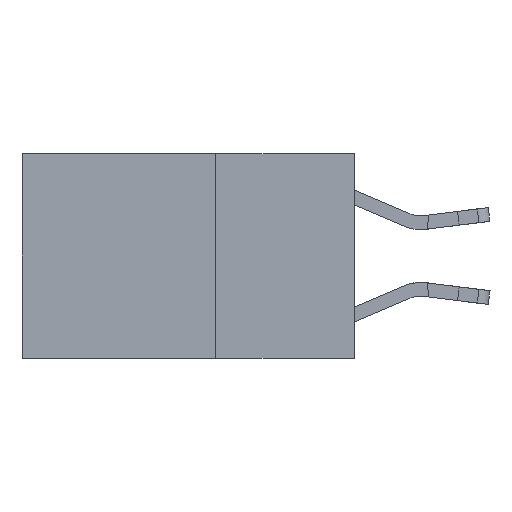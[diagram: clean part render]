
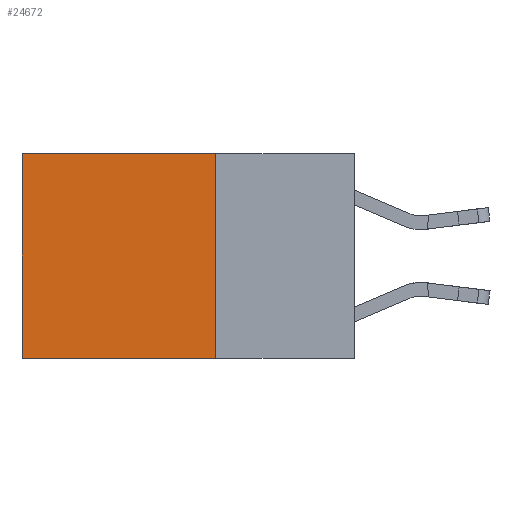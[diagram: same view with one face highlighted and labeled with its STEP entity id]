
A CAD part, left-side view. The second image highlights one B-rep face of the part: STEP entity #24672.
In plain terms, the highlighted planar face has unit normal (-1, 0, 0).
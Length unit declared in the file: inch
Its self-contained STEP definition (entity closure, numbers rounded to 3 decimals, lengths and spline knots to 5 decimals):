
#891 = CARTESIAN_POINT ( 'NONE',  ( 0.2625, 0.25, 0. ) ) ;
#1616 = CARTESIAN_POINT ( 'NONE',  ( 0.2625, 0.25, 0. ) ) ;
#2074 = ORIENTED_EDGE ( 'NONE', *, *, #21762, .F. ) ;
#2152 = LINE ( 'NONE', #8796, #12983 ) ;
#2264 = VECTOR ( 'NONE', #26236, 39.37008 ) ;
#3270 = DIRECTION ( 'NONE',  ( 0., 0., -1. ) ) ;
#4737 = CARTESIAN_POINT ( 'NONE',  ( 0.2625, 0.25, -0.37 ) ) ;
#8791 = VERTEX_POINT ( 'NONE', #13918 ) ;
#8796 = CARTESIAN_POINT ( 'NONE',  ( 0.2625, 0.25, 0. ) ) ;
#9860 = CARTESIAN_POINT ( 'NONE',  ( 0.2625, 0.25, -0.37 ) ) ;
#9944 = DIRECTION ( 'NONE',  ( 1., 0., 0. ) ) ;
#10302 = LINE ( 'NONE', #25185, #10452 ) ;
#10452 = VECTOR ( 'NONE', #3270, 39.37008 ) ;
#10700 = VERTEX_POINT ( 'NONE', #891 ) ;
#12983 = VECTOR ( 'NONE', #25919, 39.37008 ) ;
#13668 = LINE ( 'NONE', #22447, #17489 ) ;
#13902 = VERTEX_POINT ( 'NONE', #21000 ) ;
#13918 = CARTESIAN_POINT ( 'NONE',  ( 0.2625, 0.6, -0.37 ) ) ;
#14154 = EDGE_LOOP ( 'NONE', ( #15641, #2074, #20048, #23724 ) ) ;
#14256 = AXIS2_PLACEMENT_3D ( 'NONE', #1616, #9944, #18598 ) ;
#15639 = DIRECTION ( 'NONE',  ( 0., 0., -1. ) ) ;
#15641 = ORIENTED_EDGE ( 'NONE', *, *, #16255, .T. ) ;
#16255 = EDGE_CURVE ( 'NONE', #13902, #8791, #10302, .T. ) ;
#16877 = FACE_OUTER_BOUND ( 'NONE', #14154, .T. ) ;
#17441 = EDGE_CURVE ( 'NONE', #10700, #13902, #2152, .T. ) ;
#17489 = VECTOR ( 'NONE', #15639, 39.37008 ) ;
#18024 = LINE ( 'NONE', #4737, #2264 ) ;
#18598 = DIRECTION ( 'NONE',  ( 0., 0., -1. ) ) ;
#20048 = ORIENTED_EDGE ( 'NONE', *, *, #26585, .F. ) ;
#21000 = CARTESIAN_POINT ( 'NONE',  ( 0.2625, 0.6, 0. ) ) ;
#21762 = EDGE_CURVE ( 'NONE', #26251, #8791, #18024, .T. ) ;
#22447 = CARTESIAN_POINT ( 'NONE',  ( 0.2625, 0.25, 0. ) ) ;
#23724 = ORIENTED_EDGE ( 'NONE', *, *, #17441, .T. ) ;
#24672 = ADVANCED_FACE ( 'NONE', ( #16877 ), #25507, .F. ) ;
#25185 = CARTESIAN_POINT ( 'NONE',  ( 0.2625, 0.6, 0. ) ) ;
#25507 = PLANE ( 'NONE',  #14256 ) ;
#25919 = DIRECTION ( 'NONE',  ( 0., 1., 0. ) ) ;
#26236 = DIRECTION ( 'NONE',  ( 0., 1., 0. ) ) ;
#26251 = VERTEX_POINT ( 'NONE', #9860 ) ;
#26585 = EDGE_CURVE ( 'NONE', #10700, #26251, #13668, .T. ) ;
